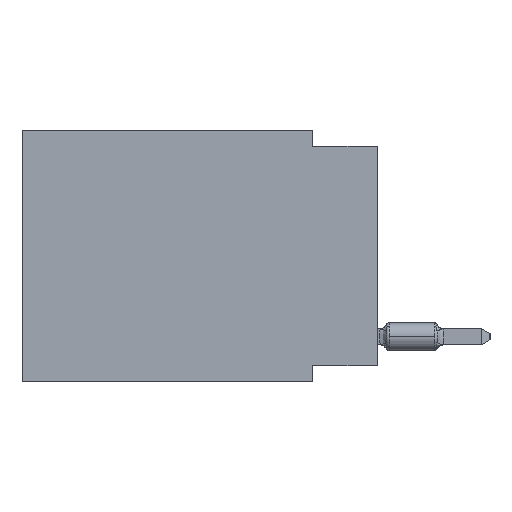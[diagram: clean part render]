
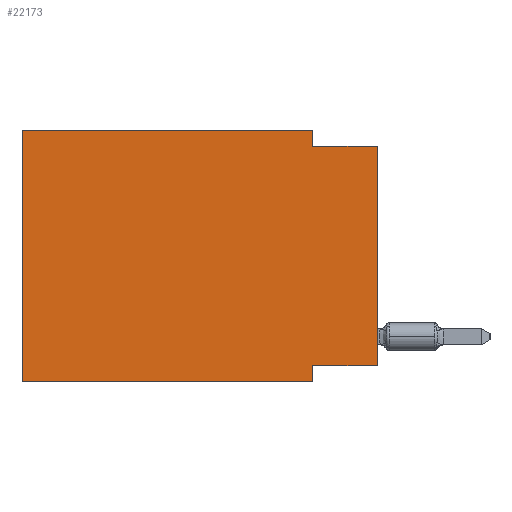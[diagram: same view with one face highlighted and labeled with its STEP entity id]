
A CAD part, left-side view. The second image highlights one B-rep face of the part: STEP entity #22173.
In plain terms, the highlighted planar face has unit normal (-1, 0, 0).
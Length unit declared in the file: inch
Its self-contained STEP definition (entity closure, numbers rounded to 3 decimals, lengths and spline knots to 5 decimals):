
#1124 = CARTESIAN_POINT ( 'NONE',  ( 0., 0., 0. ) ) ;
#1603 = VECTOR ( 'NONE', #28217, 39.37008 ) ;
#2174 = VERTEX_POINT ( 'NONE', #13734 ) ;
#2257 = ORIENTED_EDGE ( 'NONE', *, *, #16325, .F. ) ;
#2986 = VECTOR ( 'NONE', #24748, 39.37008 ) ;
#4904 = CARTESIAN_POINT ( 'NONE',  ( 0., 0.1, -0.365 ) ) ;
#5015 = LINE ( 'NONE', #1124, #1603 ) ;
#6043 = EDGE_CURVE ( 'NONE', #31213, #41171, #5015, .T. ) ;
#6219 = EDGE_CURVE ( 'NONE', #31213, #37875, #33395, .T. ) ;
#6834 = LINE ( 'NONE', #22494, #6840 ) ;
#6840 = VECTOR ( 'NONE', #7576, 39.37008 ) ;
#7576 = DIRECTION ( 'NONE',  ( 0., -1., 0. ) ) ;
#8534 = EDGE_CURVE ( 'NONE', #33222, #34797, #37086, .T. ) ;
#9644 = ORIENTED_EDGE ( 'NONE', *, *, #8534, .T. ) ;
#9725 = FACE_OUTER_BOUND ( 'NONE', #33347, .T. ) ;
#9995 = ORIENTED_EDGE ( 'NONE', *, *, #6219, .F. ) ;
#10197 = CARTESIAN_POINT ( 'NONE',  ( 0., 0.55, -0.39 ) ) ;
#11651 = ORIENTED_EDGE ( 'NONE', *, *, #6043, .T. ) ;
#12433 = VERTEX_POINT ( 'NONE', #12995 ) ;
#12995 = CARTESIAN_POINT ( 'NONE',  ( 0., 0.1, -0.025 ) ) ;
#13131 = CARTESIAN_POINT ( 'NONE',  ( 0., 0.55, 0. ) ) ;
#13457 = LINE ( 'NONE', #43106, #38640 ) ;
#13734 = CARTESIAN_POINT ( 'NONE',  ( 0., 0.1, 0. ) ) ;
#14468 = CARTESIAN_POINT ( 'NONE',  ( 0., 0.55, 0. ) ) ;
#15079 = VECTOR ( 'NONE', #48343, 39.37008 ) ;
#16325 = EDGE_CURVE ( 'NONE', #37875, #34797, #17848, .T. ) ;
#16984 = CARTESIAN_POINT ( 'NONE',  ( 0., 0.55, -0.39 ) ) ;
#17093 = AXIS2_PLACEMENT_3D ( 'NONE', #35442, #17770, #39825 ) ;
#17770 = DIRECTION ( 'NONE',  ( 1., 0., 0. ) ) ;
#17848 = LINE ( 'NONE', #44556, #46528 ) ;
#17880 = LINE ( 'NONE', #14468, #2986 ) ;
#18961 = VECTOR ( 'NONE', #43300, 39.37008 ) ;
#21036 = DIRECTION ( 'NONE',  ( 0., 0., -1. ) ) ;
#21369 = EDGE_CURVE ( 'NONE', #36631, #2174, #17880, .T. ) ;
#22085 = DIRECTION ( 'NONE',  ( 0., 1., 0. ) ) ;
#22173 = ADVANCED_FACE ( 'NONE', ( #9725 ), #43996, .F. ) ;
#22494 = CARTESIAN_POINT ( 'NONE',  ( 0., 0., -0.025 ) ) ;
#24480 = ORIENTED_EDGE ( 'NONE', *, *, #30131, .F. ) ;
#24516 = CARTESIAN_POINT ( 'NONE',  ( 0., 0.1, -0.39 ) ) ;
#24748 = DIRECTION ( 'NONE',  ( 0., -1., 0. ) ) ;
#25548 = CARTESIAN_POINT ( 'NONE',  ( 0., 0., -0.025 ) ) ;
#25902 = DIRECTION ( 'NONE',  ( 0., 0., -1. ) ) ;
#27592 = LINE ( 'NONE', #31296, #18961 ) ;
#28151 = VECTOR ( 'NONE', #22085, 39.37008 ) ;
#28217 = DIRECTION ( 'NONE',  ( 0., 0., 1. ) ) ;
#30131 = EDGE_CURVE ( 'NONE', #2174, #12433, #13457, .T. ) ;
#31213 = VERTEX_POINT ( 'NONE', #35722 ) ;
#31296 = CARTESIAN_POINT ( 'NONE',  ( 0., 0.55, 0. ) ) ;
#32538 = ORIENTED_EDGE ( 'NONE', *, *, #44637, .F. ) ;
#33222 = VERTEX_POINT ( 'NONE', #16984 ) ;
#33347 = EDGE_LOOP ( 'NONE', ( #11651, #32538, #24480, #44357, #37535, #9644, #2257, #9995 ) ) ;
#33395 = LINE ( 'NONE', #44643, #28151 ) ;
#34797 = VERTEX_POINT ( 'NONE', #24516 ) ;
#35442 = CARTESIAN_POINT ( 'NONE',  ( 0., 0.55, 0. ) ) ;
#35722 = CARTESIAN_POINT ( 'NONE',  ( 0., 0., -0.365 ) ) ;
#36631 = VERTEX_POINT ( 'NONE', #13131 ) ;
#37086 = LINE ( 'NONE', #10197, #15079 ) ;
#37535 = ORIENTED_EDGE ( 'NONE', *, *, #48330, .F. ) ;
#37875 = VERTEX_POINT ( 'NONE', #4904 ) ;
#38640 = VECTOR ( 'NONE', #21036, 39.37008 ) ;
#39825 = DIRECTION ( 'NONE',  ( 0., 0., -1. ) ) ;
#41171 = VERTEX_POINT ( 'NONE', #25548 ) ;
#43106 = CARTESIAN_POINT ( 'NONE',  ( 0., 0.1, 0. ) ) ;
#43300 = DIRECTION ( 'NONE',  ( 0., 0., 1. ) ) ;
#43996 = PLANE ( 'NONE',  #17093 ) ;
#44357 = ORIENTED_EDGE ( 'NONE', *, *, #21369, .F. ) ;
#44556 = CARTESIAN_POINT ( 'NONE',  ( 0., 0.1, -0.39 ) ) ;
#44637 = EDGE_CURVE ( 'NONE', #12433, #41171, #6834, .T. ) ;
#44643 = CARTESIAN_POINT ( 'NONE',  ( 0., 0., -0.365 ) ) ;
#46528 = VECTOR ( 'NONE', #25902, 39.37008 ) ;
#48330 = EDGE_CURVE ( 'NONE', #33222, #36631, #27592, .T. ) ;
#48343 = DIRECTION ( 'NONE',  ( 0., -1., 0. ) ) ;
